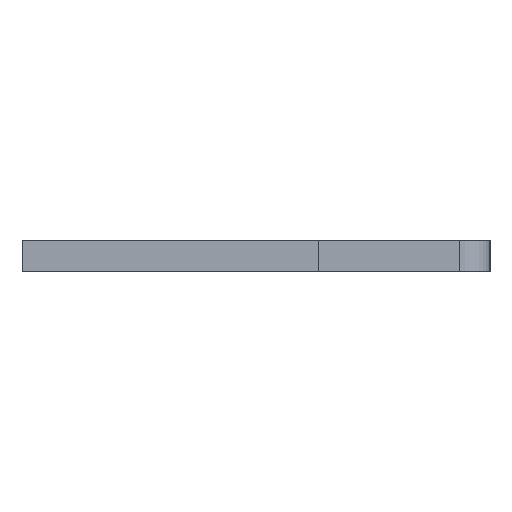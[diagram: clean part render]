
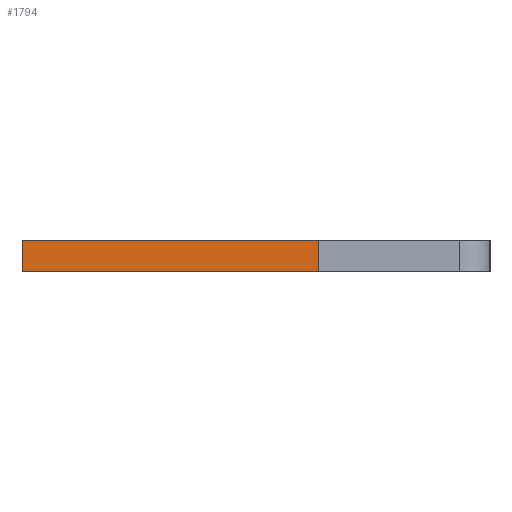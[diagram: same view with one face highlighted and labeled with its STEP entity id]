
A CAD part, left-side view. The second image highlights one B-rep face of the part: STEP entity #1794.
In plain terms, the highlighted face is planar.
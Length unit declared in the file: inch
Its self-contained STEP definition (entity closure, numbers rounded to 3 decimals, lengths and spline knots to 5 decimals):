
#61 = LINE ( 'NONE', #2388, #1165 ) ;
#103 = DIRECTION ( 'NONE',  ( -1., 0., 0. ) ) ;
#109 = VECTOR ( 'NONE', #103, 39.37008 ) ;
#148 = DIRECTION ( 'NONE',  ( 1., 0., 0. ) ) ;
#177 = DIRECTION ( 'NONE',  ( 0., 1., 0. ) ) ;
#239 = CARTESIAN_POINT ( 'NONE',  ( 0.01, 0.15, -0.04 ) ) ;
#359 = VERTEX_POINT ( 'NONE', #753 ) ;
#632 = PLANE ( 'NONE',  #3123 ) ;
#733 = VERTEX_POINT ( 'NONE', #2505 ) ;
#745 = ORIENTED_EDGE ( 'NONE', *, *, #1373, .T. ) ;
#753 = CARTESIAN_POINT ( 'NONE',  ( 0.01, -0.04, -0.04 ) ) ;
#860 = ORIENTED_EDGE ( 'NONE', *, *, #2537, .T. ) ;
#916 = EDGE_LOOP ( 'NONE', ( #860, #1536, #1245, #745 ) ) ;
#1165 = VECTOR ( 'NONE', #177, 39.37008 ) ;
#1245 = ORIENTED_EDGE ( 'NONE', *, *, #1937, .F. ) ;
#1373 = EDGE_CURVE ( 'NONE', #359, #2705, #2726, .T. ) ;
#1536 = ORIENTED_EDGE ( 'NONE', *, *, #2792, .F. ) ;
#1604 = VECTOR ( 'NONE', #2098, 39.37008 ) ;
#1794 = ADVANCED_FACE ( 'NONE', ( #2802 ), #632, .F. ) ;
#1859 = CARTESIAN_POINT ( 'NONE',  ( 0.01, 0.15, -0.04 ) ) ;
#1885 = CARTESIAN_POINT ( 'NONE',  ( 0.01, 0.15, -0.04 ) ) ;
#1937 = EDGE_CURVE ( 'NONE', #359, #733, #2818, .T. ) ;
#2098 = DIRECTION ( 'NONE',  ( -1., 0., 0. ) ) ;
#2099 = DIRECTION ( 'NONE',  ( 0., 1., 0. ) ) ;
#2182 = VECTOR ( 'NONE', #2099, 39.37008 ) ;
#2388 = CARTESIAN_POINT ( 'NONE',  ( -0.01, 0.15, -0.04 ) ) ;
#2464 = CARTESIAN_POINT ( 'NONE',  ( -0.01, 0.15, -0.04 ) ) ;
#2505 = CARTESIAN_POINT ( 'NONE',  ( 0.01, 0.15, -0.04 ) ) ;
#2537 = EDGE_CURVE ( 'NONE', #2705, #2808, #61, .T. ) ;
#2602 = DIRECTION ( 'NONE',  ( 0., 0., 1. ) ) ;
#2681 = CARTESIAN_POINT ( 'NONE',  ( -0.01, -0.04, -0.04 ) ) ;
#2705 = VERTEX_POINT ( 'NONE', #2681 ) ;
#2726 = LINE ( 'NONE', #2812, #109 ) ;
#2792 = EDGE_CURVE ( 'NONE', #733, #2808, #2986, .T. ) ;
#2802 = FACE_OUTER_BOUND ( 'NONE', #916, .T. ) ;
#2808 = VERTEX_POINT ( 'NONE', #2464 ) ;
#2812 = CARTESIAN_POINT ( 'NONE',  ( 0.01, -0.04, -0.04 ) ) ;
#2818 = LINE ( 'NONE', #1885, #2182 ) ;
#2986 = LINE ( 'NONE', #239, #1604 ) ;
#3123 = AXIS2_PLACEMENT_3D ( 'NONE', #1859, #2602, #148 ) ;
